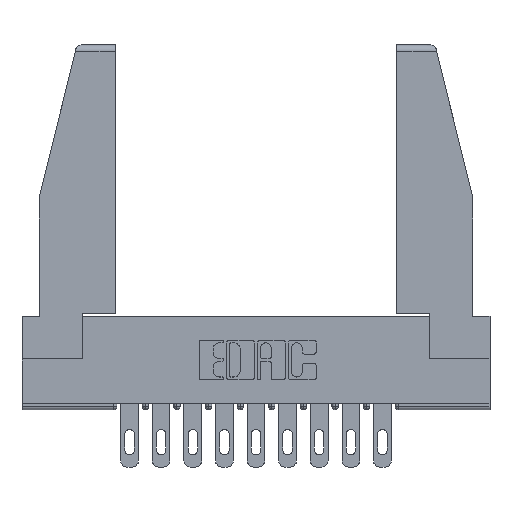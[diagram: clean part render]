
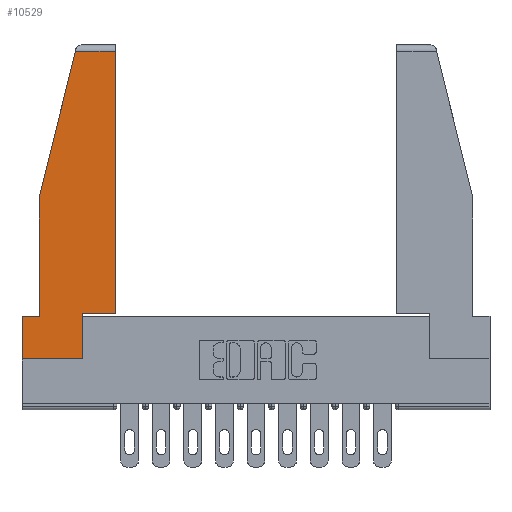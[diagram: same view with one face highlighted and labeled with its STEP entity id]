
A CAD part, top view. The second image highlights one B-rep face of the part: STEP entity #10529.
In plain terms, the highlighted planar face has unit normal (0, 0, 1).
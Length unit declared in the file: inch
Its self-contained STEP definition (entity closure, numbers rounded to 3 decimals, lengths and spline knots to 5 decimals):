
#165 = CARTESIAN_POINT ( 'NONE',  ( 0., 0., 0. ) ) ;
#287 = DIRECTION ( 'NONE',  ( -1., 0., 0. ) ) ;
#693 = CARTESIAN_POINT ( 'NONE',  ( 0.461, 0.223, 0. ) ) ;
#800 = DIRECTION ( 'NONE',  ( 1., 0., 0. ) ) ;
#884 = VERTEX_POINT ( 'NONE', #7320 ) ;
#1033 = ORIENTED_EDGE ( 'NONE', *, *, #8684, .T. ) ;
#1064 = CARTESIAN_POINT ( 'NONE',  ( 0., 1.52, 0. ) ) ;
#1341 = DIRECTION ( 'NONE',  ( 0., 0., 1. ) ) ;
#1404 = DIRECTION ( 'NONE',  ( 0., -1., 0. ) ) ;
#1474 = CARTESIAN_POINT ( 'NONE',  ( 0.297, 0.223, 0. ) ) ;
#1743 = CARTESIAN_POINT ( 'NONE',  ( 0.086, 0.8, 0. ) ) ;
#1845 = ORIENTED_EDGE ( 'NONE', *, *, #14840, .T. ) ;
#2136 = CARTESIAN_POINT ( 'NONE',  ( 0.297, 0., 0. ) ) ;
#2925 = EDGE_CURVE ( 'NONE', #7538, #9140, #13065, .T. ) ;
#2961 = VECTOR ( 'NONE', #1404, 39.37008 ) ;
#3075 = DIRECTION ( 'NONE',  ( 0., 1., 0. ) ) ;
#3889 = LINE ( 'NONE', #13336, #14822 ) ;
#4184 = LINE ( 'NONE', #693, #12899 ) ;
#4361 = LINE ( 'NONE', #11410, #4778 ) ;
#4506 = CARTESIAN_POINT ( 'NONE',  ( 0.086, 0.21, 0. ) ) ;
#4516 = CARTESIAN_POINT ( 'NONE',  ( 0., 0., 0. ) ) ;
#4748 = DIRECTION ( 'NONE',  ( 1., 0., 0. ) ) ;
#4778 = VECTOR ( 'NONE', #800, 39.37008 ) ;
#4857 = CARTESIAN_POINT ( 'NONE',  ( 0.461, 1.52, 0. ) ) ;
#4873 = LINE ( 'NONE', #14384, #14372 ) ;
#4972 = LINE ( 'NONE', #11927, #8515 ) ;
#5071 = LINE ( 'NONE', #11736, #2961 ) ;
#5435 = ORIENTED_EDGE ( 'NONE', *, *, #12984, .T. ) ;
#5732 = AXIS2_PLACEMENT_3D ( 'NONE', #165, #1341, #13039 ) ;
#6155 = DIRECTION ( 'NONE',  ( -0.239, -0.971, 0. ) ) ;
#6743 = VECTOR ( 'NONE', #12833, 39.37008 ) ;
#7320 = CARTESIAN_POINT ( 'NONE',  ( 0.461, 0.223, 0. ) ) ;
#7530 = VERTEX_POINT ( 'NONE', #1474 ) ;
#7538 = VERTEX_POINT ( 'NONE', #12310 ) ;
#8181 = FACE_OUTER_BOUND ( 'NONE', #10215, .T. ) ;
#8210 = LINE ( 'NONE', #1064, #6743 ) ;
#8461 = VERTEX_POINT ( 'NONE', #8731 ) ;
#8515 = VECTOR ( 'NONE', #4748, 39.37008 ) ;
#8684 = EDGE_CURVE ( 'NONE', #13737, #14261, #3889, .T. ) ;
#8731 = CARTESIAN_POINT ( 'NONE',  ( 0.297, 0., 0. ) ) ;
#8789 = ORIENTED_EDGE ( 'NONE', *, *, #12675, .T. ) ;
#8815 = EDGE_CURVE ( 'NONE', #14261, #12189, #5071, .T. ) ;
#9140 = VERTEX_POINT ( 'NONE', #4516 ) ;
#10054 = VERTEX_POINT ( 'NONE', #4857 ) ;
#10215 = EDGE_LOOP ( 'NONE', ( #12423, #8789, #1033, #11307, #10958, #14307, #1845, #13806, #5435 ) ) ;
#10529 = ADVANCED_FACE ( 'NONE', ( #8181 ), #10846, .T. ) ;
#10846 = PLANE ( 'NONE',  #5732 ) ;
#10925 = EDGE_CURVE ( 'NONE', #12189, #7538, #4873, .T. ) ;
#10958 = ORIENTED_EDGE ( 'NONE', *, *, #10925, .T. ) ;
#11307 = ORIENTED_EDGE ( 'NONE', *, *, #8815, .T. ) ;
#11410 = CARTESIAN_POINT ( 'NONE',  ( 0.297, 0.223, 0. ) ) ;
#11736 = CARTESIAN_POINT ( 'NONE',  ( 0.086, 0.8, 0. ) ) ;
#11927 = CARTESIAN_POINT ( 'NONE',  ( 0., 0., 0. ) ) ;
#12106 = DIRECTION ( 'NONE',  ( 0., -1., 0. ) ) ;
#12189 = VERTEX_POINT ( 'NONE', #4506 ) ;
#12191 = EDGE_CURVE ( 'NONE', #884, #10054, #4184, .T. ) ;
#12310 = CARTESIAN_POINT ( 'NONE',  ( 0., 0.21, 0. ) ) ;
#12423 = ORIENTED_EDGE ( 'NONE', *, *, #12191, .T. ) ;
#12470 = DIRECTION ( 'NONE',  ( 0., 1., 0. ) ) ;
#12675 = EDGE_CURVE ( 'NONE', #10054, #13737, #8210, .T. ) ;
#12833 = DIRECTION ( 'NONE',  ( -1., 0., 0. ) ) ;
#12899 = VECTOR ( 'NONE', #12470, 39.37008 ) ;
#12984 = EDGE_CURVE ( 'NONE', #7530, #884, #4361, .T. ) ;
#13039 = DIRECTION ( 'NONE',  ( 1., 0., 0. ) ) ;
#13065 = LINE ( 'NONE', #14219, #13362 ) ;
#13336 = CARTESIAN_POINT ( 'NONE',  ( 0.271, 1.55, 0. ) ) ;
#13362 = VECTOR ( 'NONE', #12106, 39.37008 ) ;
#13697 = LINE ( 'NONE', #2136, #14558 ) ;
#13737 = VERTEX_POINT ( 'NONE', #14983 ) ;
#13806 = ORIENTED_EDGE ( 'NONE', *, *, #15244, .T. ) ;
#14219 = CARTESIAN_POINT ( 'NONE',  ( 0., 0.21, 0. ) ) ;
#14261 = VERTEX_POINT ( 'NONE', #1743 ) ;
#14307 = ORIENTED_EDGE ( 'NONE', *, *, #2925, .T. ) ;
#14372 = VECTOR ( 'NONE', #287, 39.37008 ) ;
#14384 = CARTESIAN_POINT ( 'NONE',  ( 0., 0.21, 0. ) ) ;
#14558 = VECTOR ( 'NONE', #3075, 39.37008 ) ;
#14822 = VECTOR ( 'NONE', #6155, 39.37008 ) ;
#14840 = EDGE_CURVE ( 'NONE', #9140, #8461, #4972, .T. ) ;
#14983 = CARTESIAN_POINT ( 'NONE',  ( 0.2636, 1.52, 0. ) ) ;
#15244 = EDGE_CURVE ( 'NONE', #8461, #7530, #13697, .T. ) ;
